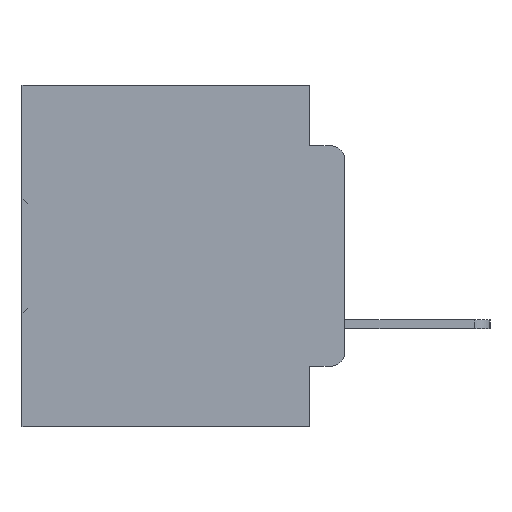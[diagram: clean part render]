
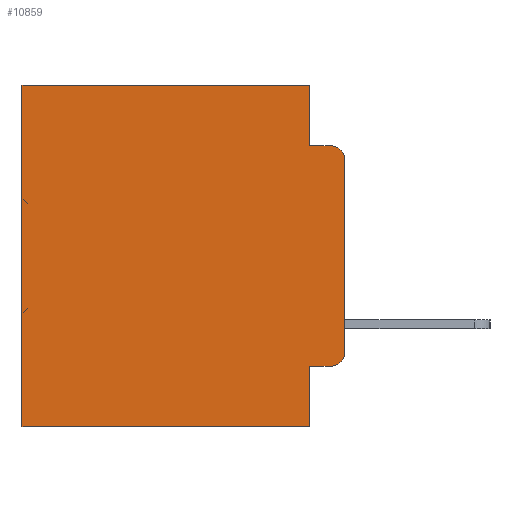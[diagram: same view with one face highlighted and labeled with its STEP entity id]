
A CAD part, left-side view. The second image highlights one B-rep face of the part: STEP entity #10859.
In plain terms, the highlighted planar face has unit normal (-1, 0, 0).
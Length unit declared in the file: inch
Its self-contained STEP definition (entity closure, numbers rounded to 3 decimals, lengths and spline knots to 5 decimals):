
#76 = CARTESIAN_POINT ( 'NONE',  ( 0.298, 0., 0. ) ) ;
#1439 = ORIENTED_EDGE ( 'NONE', *, *, #20727, .T. ) ;
#1504 = CARTESIAN_POINT ( 'NONE',  ( 0.298, 0., 0. ) ) ;
#1531 = LINE ( 'NONE', #32504, #15878 ) ;
#1778 = CARTESIAN_POINT ( 'NONE',  ( 0.298, 0., 0. ) ) ;
#2320 = VERTEX_POINT ( 'NONE', #9039 ) ;
#2639 = LINE ( 'NONE', #20700, #16880 ) ;
#2778 = CARTESIAN_POINT ( 'NONE',  ( 0.298, 0.051, 0. ) ) ;
#3078 = ORIENTED_EDGE ( 'NONE', *, *, #7868, .F. ) ;
#4102 = EDGE_CURVE ( 'NONE', #24794, #14414, #26750, .T. ) ;
#4403 = DIRECTION ( 'NONE',  ( 0., -1., 0. ) ) ;
#4670 = EDGE_CURVE ( 'NONE', #8006, #24794, #1531, .T. ) ;
#4825 = DIRECTION ( 'NONE',  ( -1., 0., 0. ) ) ;
#4919 = DIRECTION ( 'NONE',  ( 0., 0., -1. ) ) ;
#5236 = ORIENTED_EDGE ( 'NONE', *, *, #12183, .F. ) ;
#5761 = CARTESIAN_POINT ( 'NONE',  ( 0.298, 0.473, 0. ) ) ;
#5815 = ORIENTED_EDGE ( 'NONE', *, *, #10547, .T. ) ;
#7342 = VECTOR ( 'NONE', #18515, 39.37008 ) ;
#7868 = EDGE_CURVE ( 'NONE', #8006, #22584, #9154, .T. ) ;
#8006 = VERTEX_POINT ( 'NONE', #34935 ) ;
#8388 = EDGE_CURVE ( 'NONE', #11855, #2320, #2639, .T. ) ;
#8624 = CARTESIAN_POINT ( 'NONE',  ( 0.298, 0.02, -0.4115 ) ) ;
#9039 = CARTESIAN_POINT ( 'NONE',  ( 0.298, 0.473, -0.5 ) ) ;
#9154 = LINE ( 'NONE', #23764, #7342 ) ;
#9711 = CARTESIAN_POINT ( 'NONE',  ( 0.298, 0.02, -0.1085 ) ) ;
#9967 = LINE ( 'NONE', #1504, #23513 ) ;
#10547 = EDGE_CURVE ( 'NONE', #33865, #11855, #9967, .T. ) ;
#10821 = VECTOR ( 'NONE', #11103, 39.37008 ) ;
#10859 = ADVANCED_FACE ( 'NONE', ( #19728 ), #19863, .F. ) ;
#10934 = VERTEX_POINT ( 'NONE', #17656 ) ;
#11103 = DIRECTION ( 'NONE',  ( 0., 1., 0. ) ) ;
#11322 = VERTEX_POINT ( 'NONE', #35473 ) ;
#11690 = CARTESIAN_POINT ( 'NONE',  ( 0.298, 0.051, -0.5 ) ) ;
#11855 = VERTEX_POINT ( 'NONE', #5761 ) ;
#11856 = DIRECTION ( 'NONE',  ( 0., 0., -1. ) ) ;
#12183 = EDGE_CURVE ( 'NONE', #10934, #26365, #33780, .T. ) ;
#12513 = DIRECTION ( 'NONE',  ( 0., 0., -1. ) ) ;
#12609 = ORIENTED_EDGE ( 'NONE', *, *, #4670, .T. ) ;
#12909 = LINE ( 'NONE', #2778, #20869 ) ;
#13555 = VECTOR ( 'NONE', #4403, 39.37008 ) ;
#14414 = VERTEX_POINT ( 'NONE', #30698 ) ;
#14675 = EDGE_CURVE ( 'NONE', #11322, #14414, #17201, .T. ) ;
#15480 = AXIS2_PLACEMENT_3D ( 'NONE', #9711, #28489, #12513 ) ;
#15878 = VECTOR ( 'NONE', #27333, 39.37008 ) ;
#15912 = DIRECTION ( 'NONE',  ( 0., 1., 0. ) ) ;
#16541 = CARTESIAN_POINT ( 'NONE',  ( 0.298, 0.051, 0. ) ) ;
#16880 = VECTOR ( 'NONE', #23382, 39.37008 ) ;
#16964 = EDGE_CURVE ( 'NONE', #33865, #10934, #12909, .T. ) ;
#17045 = ORIENTED_EDGE ( 'NONE', *, *, #14675, .F. ) ;
#17201 = LINE ( 'NONE', #1778, #23452 ) ;
#17656 = CARTESIAN_POINT ( 'NONE',  ( 0.298, 0.051, -0.0885 ) ) ;
#18515 = DIRECTION ( 'NONE',  ( 0., 0., -1. ) ) ;
#18781 = AXIS2_PLACEMENT_3D ( 'NONE', #76, #27846, #11856 ) ;
#19256 = CARTESIAN_POINT ( 'NONE',  ( 0.298, 0., -0.5 ) ) ;
#19728 = FACE_OUTER_BOUND ( 'NONE', #35107, .T. ) ;
#19863 = PLANE ( 'NONE',  #18781 ) ;
#20700 = CARTESIAN_POINT ( 'NONE',  ( 0.298, 0.473, 0. ) ) ;
#20727 = EDGE_CURVE ( 'NONE', #11322, #26365, #32708, .T. ) ;
#20869 = VECTOR ( 'NONE', #22295, 39.37008 ) ;
#22295 = DIRECTION ( 'NONE',  ( 0., 0., -1. ) ) ;
#22367 = AXIS2_PLACEMENT_3D ( 'NONE', #28974, #4825, #28528 ) ;
#22584 = VERTEX_POINT ( 'NONE', #11690 ) ;
#23382 = DIRECTION ( 'NONE',  ( 0., 0., -1. ) ) ;
#23452 = VECTOR ( 'NONE', #4919, 39.37008 ) ;
#23513 = VECTOR ( 'NONE', #15912, 39.37008 ) ;
#23764 = CARTESIAN_POINT ( 'NONE',  ( 0.298, 0.051, 0. ) ) ;
#23797 = CARTESIAN_POINT ( 'NONE',  ( 0.298, 0.02, -0.0885 ) ) ;
#24335 = ORIENTED_EDGE ( 'NONE', *, *, #26637, .F. ) ;
#24794 = VERTEX_POINT ( 'NONE', #8624 ) ;
#25130 = LINE ( 'NONE', #19256, #10821 ) ;
#26365 = VERTEX_POINT ( 'NONE', #23797 ) ;
#26395 = CARTESIAN_POINT ( 'NONE',  ( 0.298, 0.051, -0.0885 ) ) ;
#26637 = EDGE_CURVE ( 'NONE', #22584, #2320, #25130, .T. ) ;
#26750 = CIRCLE ( 'NONE', #22367, 0.02 ) ;
#27333 = DIRECTION ( 'NONE',  ( 0., -1., 0. ) ) ;
#27846 = DIRECTION ( 'NONE',  ( 1., 0., 0. ) ) ;
#28489 = DIRECTION ( 'NONE',  ( -1., 0., 0. ) ) ;
#28528 = DIRECTION ( 'NONE',  ( 0., 0., -1. ) ) ;
#28974 = CARTESIAN_POINT ( 'NONE',  ( 0.298, 0.02, -0.3915 ) ) ;
#29559 = ORIENTED_EDGE ( 'NONE', *, *, #16964, .F. ) ;
#30466 = ORIENTED_EDGE ( 'NONE', *, *, #4102, .T. ) ;
#30698 = CARTESIAN_POINT ( 'NONE',  ( 0.298, 0., -0.3915 ) ) ;
#32504 = CARTESIAN_POINT ( 'NONE',  ( 0.298, 0.051, -0.4115 ) ) ;
#32708 = CIRCLE ( 'NONE', #15480, 0.02 ) ;
#33780 = LINE ( 'NONE', #26395, #13555 ) ;
#33865 = VERTEX_POINT ( 'NONE', #16541 ) ;
#34935 = CARTESIAN_POINT ( 'NONE',  ( 0.298, 0.051, -0.4115 ) ) ;
#35107 = EDGE_LOOP ( 'NONE', ( #17045, #1439, #5236, #29559, #5815, #35342, #24335, #3078, #12609, #30466 ) ) ;
#35342 = ORIENTED_EDGE ( 'NONE', *, *, #8388, .T. ) ;
#35473 = CARTESIAN_POINT ( 'NONE',  ( 0.298, 0., -0.1085 ) ) ;
